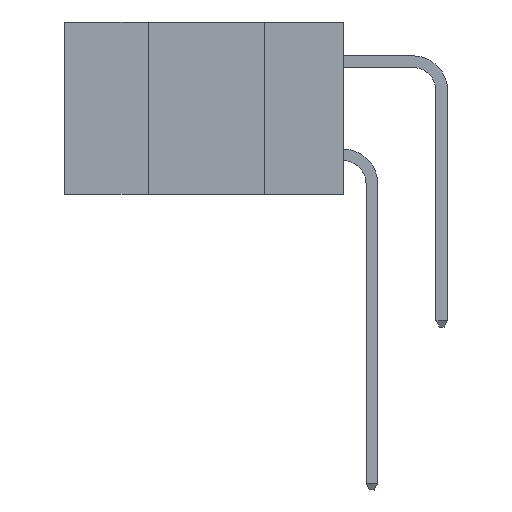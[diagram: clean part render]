
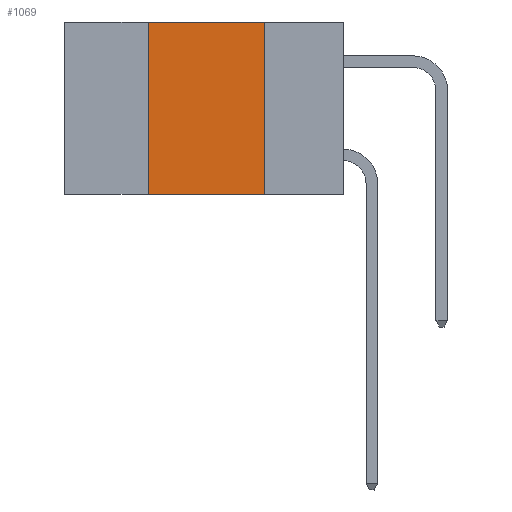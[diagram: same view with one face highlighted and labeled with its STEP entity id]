
A CAD part, left-side view. The second image highlights one B-rep face of the part: STEP entity #1069.
In plain terms, the highlighted planar face has unit normal (-1, 0, 0).
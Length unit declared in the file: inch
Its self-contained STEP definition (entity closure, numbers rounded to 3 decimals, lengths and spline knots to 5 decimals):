
#242 = DIRECTION ( 'NONE',  ( 1., 0., 0. ) ) ;
#398 = LINE ( 'NONE', #6550, #2750 ) ;
#478 = EDGE_LOOP ( 'NONE', ( #1085, #3302, #11742, #5528 ) ) ;
#685 = LINE ( 'NONE', #4411, #5664 ) ;
#1069 = ADVANCED_FACE ( 'NONE', ( #7007 ), #3225, .F. ) ;
#1085 = ORIENTED_EDGE ( 'NONE', *, *, #6320, .F. ) ;
#1187 = CARTESIAN_POINT ( 'NONE',  ( 0., 0.17, -0.37 ) ) ;
#1451 = VERTEX_POINT ( 'NONE', #2868 ) ;
#1653 = AXIS2_PLACEMENT_3D ( 'NONE', #4759, #242, #12517 ) ;
#1806 = EDGE_CURVE ( 'NONE', #2142, #8267, #11315, .T. ) ;
#2142 = VERTEX_POINT ( 'NONE', #4356 ) ;
#2750 = VECTOR ( 'NONE', #2972, 39.37008 ) ;
#2868 = CARTESIAN_POINT ( 'NONE',  ( 0., 0.17, 0. ) ) ;
#2972 = DIRECTION ( 'NONE',  ( 0., -1., 0. ) ) ;
#3224 = DIRECTION ( 'NONE',  ( 0., 0., -1. ) ) ;
#3225 = PLANE ( 'NONE',  #1653 ) ;
#3302 = ORIENTED_EDGE ( 'NONE', *, *, #4768, .F. ) ;
#4356 = CARTESIAN_POINT ( 'NONE',  ( 0., 0.42, -0.37 ) ) ;
#4411 = CARTESIAN_POINT ( 'NONE',  ( 0., 0.17, 0. ) ) ;
#4753 = VERTEX_POINT ( 'NONE', #10266 ) ;
#4759 = CARTESIAN_POINT ( 'NONE',  ( 0., 0.6, 0. ) ) ;
#4768 = EDGE_CURVE ( 'NONE', #4753, #1451, #398, .T. ) ;
#5528 = ORIENTED_EDGE ( 'NONE', *, *, #1806, .T. ) ;
#5664 = VECTOR ( 'NONE', #3224, 39.37008 ) ;
#5951 = EDGE_CURVE ( 'NONE', #2142, #4753, #11922, .T. ) ;
#6320 = EDGE_CURVE ( 'NONE', #1451, #8267, #685, .T. ) ;
#6550 = CARTESIAN_POINT ( 'NONE',  ( 0., 0.6, 0. ) ) ;
#7007 = FACE_OUTER_BOUND ( 'NONE', #478, .T. ) ;
#7037 = CARTESIAN_POINT ( 'NONE',  ( 0., 0.6, -0.37 ) ) ;
#7241 = DIRECTION ( 'NONE',  ( 0., -1., 0. ) ) ;
#8267 = VERTEX_POINT ( 'NONE', #1187 ) ;
#9152 = VECTOR ( 'NONE', #7241, 39.37008 ) ;
#10266 = CARTESIAN_POINT ( 'NONE',  ( 0., 0.42, 0. ) ) ;
#10628 = DIRECTION ( 'NONE',  ( 0., 0., 1. ) ) ;
#10648 = CARTESIAN_POINT ( 'NONE',  ( 0., 0.42, 0. ) ) ;
#11315 = LINE ( 'NONE', #7037, #9152 ) ;
#11607 = VECTOR ( 'NONE', #10628, 39.37008 ) ;
#11742 = ORIENTED_EDGE ( 'NONE', *, *, #5951, .F. ) ;
#11922 = LINE ( 'NONE', #10648, #11607 ) ;
#12517 = DIRECTION ( 'NONE',  ( 0., 0., -1. ) ) ;
